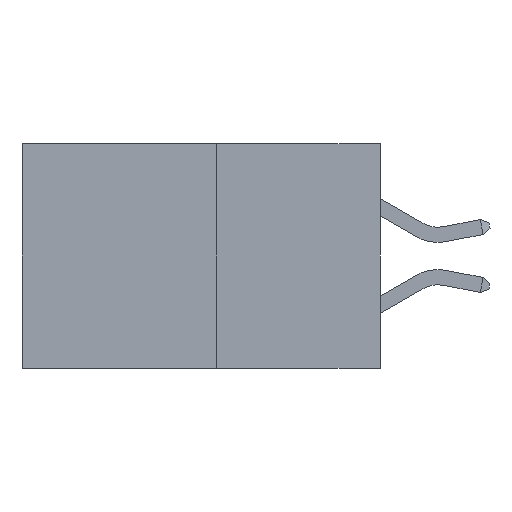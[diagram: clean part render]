
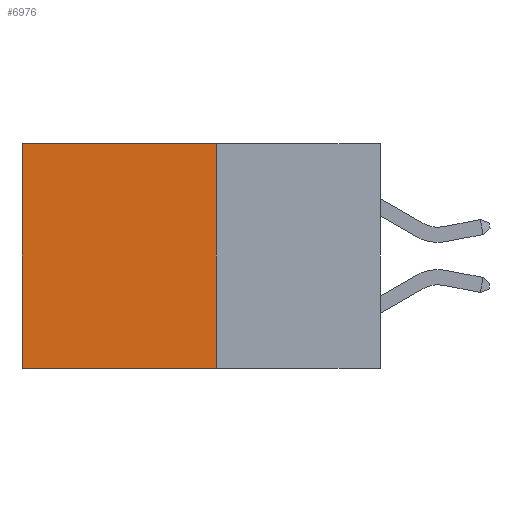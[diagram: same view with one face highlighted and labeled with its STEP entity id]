
A CAD part, left-side view. The second image highlights one B-rep face of the part: STEP entity #6976.
In plain terms, the highlighted planar face has unit normal (-1, 0, 0).
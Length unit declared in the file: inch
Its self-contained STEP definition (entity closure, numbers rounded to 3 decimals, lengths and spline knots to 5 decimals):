
#174 = DIRECTION ( 'NONE',  ( 0., 1., 0. ) ) ;
#390 = EDGE_CURVE ( 'NONE', #1177, #1108, #7302, .T. ) ;
#476 = DIRECTION ( 'NONE',  ( 1., 0., 0. ) ) ;
#706 = CARTESIAN_POINT ( 'NONE',  ( 0.277, 0.27, 0. ) ) ;
#1009 = DIRECTION ( 'NONE',  ( 0., 0., -1. ) ) ;
#1047 = ORIENTED_EDGE ( 'NONE', *, *, #390, .F. ) ;
#1108 = VERTEX_POINT ( 'NONE', #6145 ) ;
#1177 = VERTEX_POINT ( 'NONE', #3626 ) ;
#1996 = CARTESIAN_POINT ( 'NONE',  ( 0.277, 0.27, -0.37 ) ) ;
#2413 = CARTESIAN_POINT ( 'NONE',  ( 0.277, 0.59, 0. ) ) ;
#3031 = VECTOR ( 'NONE', #7120, 39.37008 ) ;
#3480 = ORIENTED_EDGE ( 'NONE', *, *, #7660, .T. ) ;
#3585 = CARTESIAN_POINT ( 'NONE',  ( 0.277, 0.59, -0.37 ) ) ;
#3626 = CARTESIAN_POINT ( 'NONE',  ( 0.277, 0.27, -0.37 ) ) ;
#3692 = VERTEX_POINT ( 'NONE', #8850 ) ;
#4233 = VECTOR ( 'NONE', #1009, 39.37008 ) ;
#4589 = VECTOR ( 'NONE', #9133, 39.37008 ) ;
#4924 = EDGE_LOOP ( 'NONE', ( #3480, #1047, #6696, #8829 ) ) ;
#5312 = LINE ( 'NONE', #3585, #3031 ) ;
#5348 = AXIS2_PLACEMENT_3D ( 'NONE', #1996, #476, #5516 ) ;
#5516 = DIRECTION ( 'NONE',  ( 0., 0., -1. ) ) ;
#5822 = VECTOR ( 'NONE', #174, 39.37008 ) ;
#5956 = CARTESIAN_POINT ( 'NONE',  ( 0.277, 0.27, -0.37 ) ) ;
#6032 = EDGE_CURVE ( 'NONE', #3692, #7303, #6449, .T. ) ;
#6067 = LINE ( 'NONE', #5956, #4233 ) ;
#6145 = CARTESIAN_POINT ( 'NONE',  ( 0.277, 0.59, -0.37 ) ) ;
#6299 = FACE_OUTER_BOUND ( 'NONE', #4924, .T. ) ;
#6449 = LINE ( 'NONE', #706, #4589 ) ;
#6696 = ORIENTED_EDGE ( 'NONE', *, *, #7393, .F. ) ;
#6976 = ADVANCED_FACE ( 'NONE', ( #6299 ), #7659, .F. ) ;
#7120 = DIRECTION ( 'NONE',  ( 0., 0., -1. ) ) ;
#7302 = LINE ( 'NONE', #7417, #5822 ) ;
#7303 = VERTEX_POINT ( 'NONE', #2413 ) ;
#7393 = EDGE_CURVE ( 'NONE', #3692, #1177, #6067, .T. ) ;
#7417 = CARTESIAN_POINT ( 'NONE',  ( 0.277, 0.27, -0.37 ) ) ;
#7659 = PLANE ( 'NONE',  #5348 ) ;
#7660 = EDGE_CURVE ( 'NONE', #7303, #1108, #5312, .T. ) ;
#8829 = ORIENTED_EDGE ( 'NONE', *, *, #6032, .T. ) ;
#8850 = CARTESIAN_POINT ( 'NONE',  ( 0.277, 0.27, 0. ) ) ;
#9133 = DIRECTION ( 'NONE',  ( 0., 1., 0. ) ) ;
